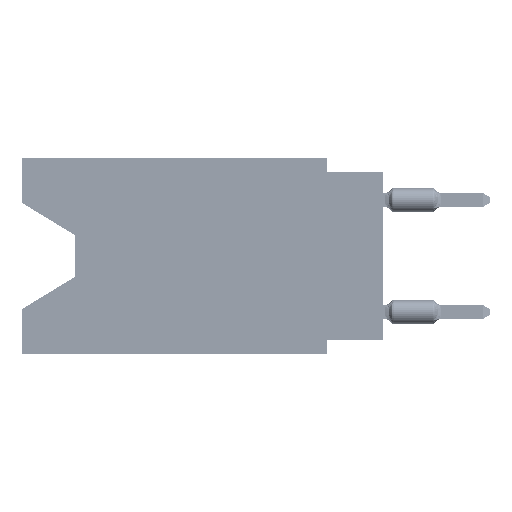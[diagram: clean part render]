
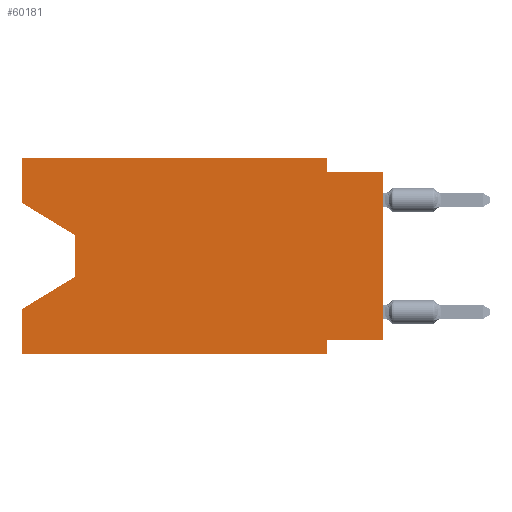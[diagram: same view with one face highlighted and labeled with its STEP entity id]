
A CAD part, left-side view. The second image highlights one B-rep face of the part: STEP entity #60181.
In plain terms, the highlighted planar face has unit normal (-1, 0, 0).
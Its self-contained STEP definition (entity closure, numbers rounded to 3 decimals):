
#2251 = LINE ( 'NONE', #68264, #23372 ) ;
#3741 = EDGE_CURVE ( 'NONE', #77662, #78113, #2251, .T. ) ;
#4415 = LINE ( 'NONE', #28441, #34726 ) ;
#4422 = EDGE_CURVE ( 'NONE', #34519, #77606, #20513, .T. ) ;
#5240 = VECTOR ( 'NONE', #38585, 1000. ) ;
#6348 = DIRECTION ( 'NONE',  ( 1., 0., 0. ) ) ;
#7386 = LINE ( 'NONE', #22123, #28835 ) ;
#7766 = EDGE_CURVE ( 'NONE', #34519, #71050, #64768, .T. ) ;
#9385 = ORIENTED_EDGE ( 'NONE', *, *, #57312, .F. ) ;
#10141 = VERTEX_POINT ( 'NONE', #16937 ) ;
#10784 = ORIENTED_EDGE ( 'NONE', *, *, #3741, .F. ) ;
#11655 = CARTESIAN_POINT ( 'NONE',  ( 0., 2.54, -0.635 ) ) ;
#12089 = ORIENTED_EDGE ( 'NONE', *, *, #17194, .F. ) ;
#12380 = EDGE_CURVE ( 'NONE', #91941, #57067, #31860, .T. ) ;
#12550 = DIRECTION ( 'NONE',  ( 0., 0., -1. ) ) ;
#13163 = CARTESIAN_POINT ( 'NONE',  ( 0., 16.383, -8.89 ) ) ;
#13649 = VECTOR ( 'NONE', #92957, 1000. ) ;
#14472 = DIRECTION ( 'NONE',  ( 0., 0., -1. ) ) ;
#14528 = CARTESIAN_POINT ( 'NONE',  ( 0., 16.383, 0. ) ) ;
#15190 = CARTESIAN_POINT ( 'NONE',  ( 0., 13.97, -3.505 ) ) ;
#16051 = EDGE_CURVE ( 'NONE', #91941, #10141, #21131, .T. ) ;
#16937 = CARTESIAN_POINT ( 'NONE',  ( 0., 16.383, 0. ) ) ;
#17136 = ORIENTED_EDGE ( 'NONE', *, *, #70647, .F. ) ;
#17194 = EDGE_CURVE ( 'NONE', #77606, #48965, #38186, .T. ) ;
#20513 = LINE ( 'NONE', #88667, #49866 ) ;
#20581 = ORIENTED_EDGE ( 'NONE', *, *, #86975, .T. ) ;
#21131 = LINE ( 'NONE', #72378, #94918 ) ;
#22123 = CARTESIAN_POINT ( 'NONE',  ( 0., 13.97, -3.505 ) ) ;
#23372 = VECTOR ( 'NONE', #85717, 1000. ) ;
#26133 = DIRECTION ( 'NONE',  ( 0., -1., 0. ) ) ;
#26275 = VERTEX_POINT ( 'NONE', #87359 ) ;
#26947 = CARTESIAN_POINT ( 'NONE',  ( 0., 0., -0.635 ) ) ;
#28441 = CARTESIAN_POINT ( 'NONE',  ( 0., 0., -0.635 ) ) ;
#28469 = DIRECTION ( 'NONE',  ( 0., -1., 0. ) ) ;
#28835 = VECTOR ( 'NONE', #14472, 1000. ) ;
#30782 = DIRECTION ( 'NONE',  ( 0., -0.855, -0.519 ) ) ;
#30923 = DIRECTION ( 'NONE',  ( 0., 0., 1. ) ) ;
#31860 = LINE ( 'NONE', #56403, #38654 ) ;
#32029 = CARTESIAN_POINT ( 'NONE',  ( 0., 2.54, -8.89 ) ) ;
#34105 = VECTOR ( 'NONE', #12550, 1000. ) ;
#34519 = VERTEX_POINT ( 'NONE', #100531 ) ;
#34607 = EDGE_CURVE ( 'NONE', #86367, #48965, #69396, .T. ) ;
#34726 = VECTOR ( 'NONE', #47486, 1000. ) ;
#34865 = CARTESIAN_POINT ( 'NONE',  ( 0., 2.54, -8.255 ) ) ;
#35283 = EDGE_LOOP ( 'NONE', ( #48413, #20581, #73511, #103883, #69054, #12089, #35593, #84514, #9385, #10784, #17136, #56707 ) ) ;
#35593 = ORIENTED_EDGE ( 'NONE', *, *, #4422, .F. ) ;
#35974 = LINE ( 'NONE', #52334, #63898 ) ;
#38186 = LINE ( 'NONE', #32029, #34105 ) ;
#38585 = DIRECTION ( 'NONE',  ( 0., 0., 1. ) ) ;
#38654 = VECTOR ( 'NONE', #30782, 1000. ) ;
#42502 = CARTESIAN_POINT ( 'NONE',  ( 0., 2.54, 0. ) ) ;
#43778 = VECTOR ( 'NONE', #28469, 1000. ) ;
#44111 = CARTESIAN_POINT ( 'NONE',  ( 0., 16.383, 0. ) ) ;
#46401 = VERTEX_POINT ( 'NONE', #106297 ) ;
#47198 = DIRECTION ( 'NONE',  ( 0., 1., 0. ) ) ;
#47486 = DIRECTION ( 'NONE',  ( 0., -1., 0. ) ) ;
#48413 = ORIENTED_EDGE ( 'NONE', *, *, #12380, .T. ) ;
#48965 = VERTEX_POINT ( 'NONE', #77355 ) ;
#49866 = VECTOR ( 'NONE', #47198, 1000. ) ;
#52334 = CARTESIAN_POINT ( 'NONE',  ( 0., 16.383, 0. ) ) ;
#54845 = CARTESIAN_POINT ( 'NONE',  ( 0., 16.383, -2.038 ) ) ;
#55513 = CARTESIAN_POINT ( 'NONE',  ( 0., 16.383, -8.89 ) ) ;
#56403 = CARTESIAN_POINT ( 'NONE',  ( 0., 16.383, -2.038 ) ) ;
#56518 = DIRECTION ( 'NONE',  ( 0., 0., -1. ) ) ;
#56707 = ORIENTED_EDGE ( 'NONE', *, *, #16051, .F. ) ;
#57067 = VERTEX_POINT ( 'NONE', #15190 ) ;
#57312 = EDGE_CURVE ( 'NONE', #78113, #71050, #4415, .T. ) ;
#60181 = ADVANCED_FACE ( 'NONE', ( #89277 ), #64721, .F. ) ;
#63898 = VECTOR ( 'NONE', #75818, 1000. ) ;
#64721 = PLANE ( 'NONE',  #90649 ) ;
#64768 = LINE ( 'NONE', #98044, #5240 ) ;
#64874 = EDGE_CURVE ( 'NONE', #86367, #26275, #35974, .T. ) ;
#68264 = CARTESIAN_POINT ( 'NONE',  ( 0., 2.54, 0. ) ) ;
#68576 = EDGE_CURVE ( 'NONE', #46401, #26275, #101140, .T. ) ;
#69054 = ORIENTED_EDGE ( 'NONE', *, *, #34607, .T. ) ;
#69396 = LINE ( 'NONE', #13163, #43778 ) ;
#70647 = EDGE_CURVE ( 'NONE', #10141, #77662, #106362, .T. ) ;
#71050 = VERTEX_POINT ( 'NONE', #26947 ) ;
#72378 = CARTESIAN_POINT ( 'NONE',  ( 0., 16.383, 0. ) ) ;
#73511 = ORIENTED_EDGE ( 'NONE', *, *, #68576, .T. ) ;
#75818 = DIRECTION ( 'NONE',  ( 0., 0., 1. ) ) ;
#77355 = CARTESIAN_POINT ( 'NONE',  ( 0., 2.54, -8.89 ) ) ;
#77606 = VERTEX_POINT ( 'NONE', #34865 ) ;
#77662 = VERTEX_POINT ( 'NONE', #42502 ) ;
#78113 = VERTEX_POINT ( 'NONE', #11655 ) ;
#84514 = ORIENTED_EDGE ( 'NONE', *, *, #7766, .T. ) ;
#85717 = DIRECTION ( 'NONE',  ( 0., 0., -1. ) ) ;
#86367 = VERTEX_POINT ( 'NONE', #55513 ) ;
#86975 = EDGE_CURVE ( 'NONE', #57067, #46401, #7386, .T. ) ;
#87359 = CARTESIAN_POINT ( 'NONE',  ( 0., 16.383, -6.852 ) ) ;
#88667 = CARTESIAN_POINT ( 'NONE',  ( 0., 0., -8.255 ) ) ;
#89277 = FACE_OUTER_BOUND ( 'NONE', #35283, .T. ) ;
#90649 = AXIS2_PLACEMENT_3D ( 'NONE', #14528, #6348, #56518 ) ;
#91941 = VERTEX_POINT ( 'NONE', #54845 ) ;
#92957 = DIRECTION ( 'NONE',  ( 0., 0.855, -0.519 ) ) ;
#94105 = VECTOR ( 'NONE', #26133, 1000. ) ;
#94918 = VECTOR ( 'NONE', #30923, 1000. ) ;
#98044 = CARTESIAN_POINT ( 'NONE',  ( 0., 0., 0. ) ) ;
#100531 = CARTESIAN_POINT ( 'NONE',  ( 0., 0., -8.255 ) ) ;
#100610 = CARTESIAN_POINT ( 'NONE',  ( 0., 13.97, -5.385 ) ) ;
#101140 = LINE ( 'NONE', #100610, #13649 ) ;
#103883 = ORIENTED_EDGE ( 'NONE', *, *, #64874, .F. ) ;
#106297 = CARTESIAN_POINT ( 'NONE',  ( 0., 13.97, -5.385 ) ) ;
#106362 = LINE ( 'NONE', #44111, #94105 ) ;
